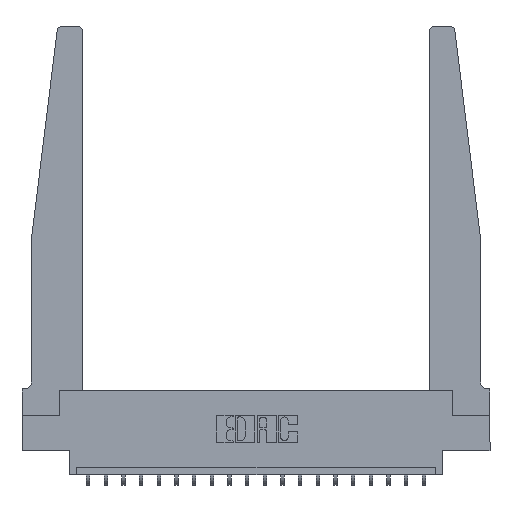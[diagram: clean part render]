
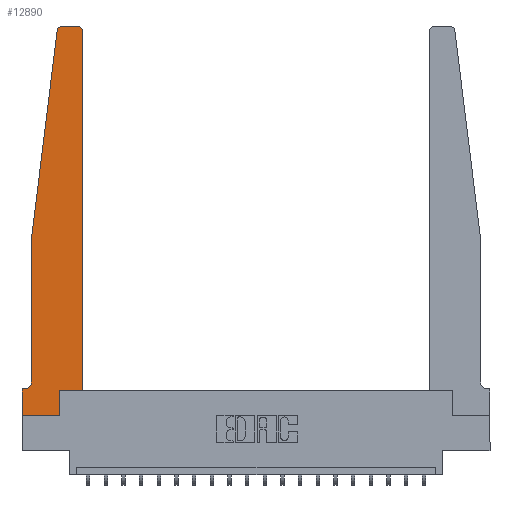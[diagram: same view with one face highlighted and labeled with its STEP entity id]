
A CAD part, top view. The second image highlights one B-rep face of the part: STEP entity #12890.
In plain terms, the highlighted planar face has unit normal (0, 0, 1).
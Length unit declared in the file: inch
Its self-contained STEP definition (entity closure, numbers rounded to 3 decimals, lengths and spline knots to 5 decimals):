
#287 = VECTOR ( 'NONE', #11607, 39.37008 ) ;
#391 = EDGE_CURVE ( 'NONE', #1555, #17705, #18310, .T. ) ;
#419 = LINE ( 'NONE', #6538, #4378 ) ;
#451 = DIRECTION ( 'NONE',  ( -1., 0., 0. ) ) ;
#769 = CARTESIAN_POINT ( 'NONE',  ( 0.395, 2.72, 0.37 ) ) ;
#806 = CARTESIAN_POINT ( 'NONE',  ( 0.2605, 0.18, 0.37 ) ) ;
#809 = EDGE_CURVE ( 'NONE', #17705, #7202, #2419, .T. ) ;
#1295 = LINE ( 'NONE', #3190, #1606 ) ;
#1555 = VERTEX_POINT ( 'NONE', #19395 ) ;
#1606 = VECTOR ( 'NONE', #17604, 39.37008 ) ;
#1727 = CARTESIAN_POINT ( 'NONE',  ( 0., 0.1875, 0.37 ) ) ;
#1750 = CARTESIAN_POINT ( 'NONE',  ( 0.015, 0.1875, 0.37 ) ) ;
#1813 = ORIENTED_EDGE ( 'NONE', *, *, #809, .T. ) ;
#2112 = DIRECTION ( 'NONE',  ( -1., 0., 0. ) ) ;
#2259 = CARTESIAN_POINT ( 'NONE',  ( 0.425, 2.72, 0.37 ) ) ;
#2419 = LINE ( 'NONE', #16705, #19772 ) ;
#3012 = EDGE_LOOP ( 'NONE', ( #16483, #19728, #16349, #1813, #17590, #5781, #17220, #20670, #18151, #8635, #3396, #18256 ) ) ;
#3190 = CARTESIAN_POINT ( 'NONE',  ( 0., 0., 0.37 ) ) ;
#3396 = ORIENTED_EDGE ( 'NONE', *, *, #15649, .T. ) ;
#3664 = CARTESIAN_POINT ( 'NONE',  ( 0.425, 0.18, 0.37 ) ) ;
#3763 = DIRECTION ( 'NONE',  ( 0., 0., 1. ) ) ;
#3766 = VERTEX_POINT ( 'NONE', #19923 ) ;
#4326 = DIRECTION ( 'NONE',  ( 0., 1., 0. ) ) ;
#4370 = CARTESIAN_POINT ( 'NONE',  ( 0.2605, 0.18, 0.37 ) ) ;
#4378 = VECTOR ( 'NONE', #2112, 39.37008 ) ;
#4494 = CARTESIAN_POINT ( 'NONE',  ( 0.015, 0.2375, 0.37 ) ) ;
#4539 = AXIS2_PLACEMENT_3D ( 'NONE', #9388, #11543, #19548 ) ;
#4913 = VERTEX_POINT ( 'NONE', #15503 ) ;
#4918 = VECTOR ( 'NONE', #8420, 39.37008 ) ;
#5444 = EDGE_CURVE ( 'NONE', #6255, #16433, #419, .T. ) ;
#5508 = CARTESIAN_POINT ( 'NONE',  ( 0.065, 1.25, 0.37 ) ) ;
#5580 = LINE ( 'NONE', #15124, #4918 ) ;
#5781 = ORIENTED_EDGE ( 'NONE', *, *, #5444, .T. ) ;
#5790 = VECTOR ( 'NONE', #8516, 39.37008 ) ;
#5937 = EDGE_CURVE ( 'NONE', #8788, #1555, #10080, .T. ) ;
#6122 = LINE ( 'NONE', #10741, #7025 ) ;
#6255 = VERTEX_POINT ( 'NONE', #1750 ) ;
#6275 = CARTESIAN_POINT ( 'NONE',  ( 0.065, 1.25, 0.37 ) ) ;
#6538 = CARTESIAN_POINT ( 'NONE',  ( 0.065, 0.1875, 0.37 ) ) ;
#6675 = EDGE_CURVE ( 'NONE', #16186, #20377, #12106, .T. ) ;
#6851 = FACE_OUTER_BOUND ( 'NONE', #3012, .T. ) ;
#7025 = VECTOR ( 'NONE', #4326, 39.37008 ) ;
#7202 = VERTEX_POINT ( 'NONE', #18635 ) ;
#7243 = CARTESIAN_POINT ( 'NONE',  ( 0.27653, 2.72, 0.37 ) ) ;
#7995 = EDGE_CURVE ( 'NONE', #12385, #4913, #18066, .T. ) ;
#8420 = DIRECTION ( 'NONE',  ( 0., -1., 0. ) ) ;
#8437 = CARTESIAN_POINT ( 'NONE',  ( 0.395, 2.75, 0.37 ) ) ;
#8516 = DIRECTION ( 'NONE',  ( 1., 0., 0. ) ) ;
#8635 = ORIENTED_EDGE ( 'NONE', *, *, #7995, .T. ) ;
#8788 = VERTEX_POINT ( 'NONE', #18329 ) ;
#9281 = CARTESIAN_POINT ( 'NONE',  ( 0.2605, 0., 0.37 ) ) ;
#9388 = CARTESIAN_POINT ( 'NONE',  ( 0., 0.1875, 0.37 ) ) ;
#10080 = CIRCLE ( 'NONE', #18142, 0.03 ) ;
#10436 = DIRECTION ( 'NONE',  ( -0.122, -0.992, 0. ) ) ;
#10741 = CARTESIAN_POINT ( 'NONE',  ( 0.425, 0.18, 0.37 ) ) ;
#11082 = VERTEX_POINT ( 'NONE', #9281 ) ;
#11543 = DIRECTION ( 'NONE',  ( 0., 0., 1. ) ) ;
#11607 = DIRECTION ( 'NONE',  ( -1., 0., 0. ) ) ;
#11664 = VECTOR ( 'NONE', #10436, 39.37008 ) ;
#11689 = DIRECTION ( 'NONE',  ( 0., 0., 1. ) ) ;
#12106 = CIRCLE ( 'NONE', #16835, 0.03 ) ;
#12385 = VERTEX_POINT ( 'NONE', #4370 ) ;
#12890 = ADVANCED_FACE ( 'NONE', ( #6851 ), #19751, .T. ) ;
#13372 = DIRECTION ( 'NONE',  ( 1., 0., 0. ) ) ;
#13417 = EDGE_CURVE ( 'NONE', #11082, #12385, #19724, .T. ) ;
#13548 = DIRECTION ( 'NONE',  ( 0., -1., 0. ) ) ;
#14740 = EDGE_CURVE ( 'NONE', #16433, #3766, #5580, .T. ) ;
#15124 = CARTESIAN_POINT ( 'NONE',  ( 0., 0., 0.37 ) ) ;
#15503 = CARTESIAN_POINT ( 'NONE',  ( 0.425, 0.18, 0.37 ) ) ;
#15649 = EDGE_CURVE ( 'NONE', #4913, #16186, #6122, .T. ) ;
#16146 = LINE ( 'NONE', #19300, #287 ) ;
#16186 = VERTEX_POINT ( 'NONE', #2259 ) ;
#16349 = ORIENTED_EDGE ( 'NONE', *, *, #391, .T. ) ;
#16433 = VERTEX_POINT ( 'NONE', #1727 ) ;
#16483 = ORIENTED_EDGE ( 'NONE', *, *, #17805, .T. ) ;
#16542 = EDGE_CURVE ( 'NONE', #3766, #11082, #1295, .T. ) ;
#16705 = CARTESIAN_POINT ( 'NONE',  ( 0.065, 1.25, 0.37 ) ) ;
#16835 = AXIS2_PLACEMENT_3D ( 'NONE', #769, #11689, #13372 ) ;
#17220 = ORIENTED_EDGE ( 'NONE', *, *, #14740, .T. ) ;
#17307 = DIRECTION ( 'NONE',  ( 0., 0., -1. ) ) ;
#17590 = ORIENTED_EDGE ( 'NONE', *, *, #19909, .T. ) ;
#17604 = DIRECTION ( 'NONE',  ( 1., 0., 0. ) ) ;
#17705 = VERTEX_POINT ( 'NONE', #6275 ) ;
#17805 = EDGE_CURVE ( 'NONE', #20377, #8788, #16146, .T. ) ;
#17981 = VECTOR ( 'NONE', #20039, 39.37008 ) ;
#18066 = LINE ( 'NONE', #3664, #5790 ) ;
#18142 = AXIS2_PLACEMENT_3D ( 'NONE', #7243, #3763, #19950 ) ;
#18151 = ORIENTED_EDGE ( 'NONE', *, *, #13417, .T. ) ;
#18256 = ORIENTED_EDGE ( 'NONE', *, *, #6675, .T. ) ;
#18310 = LINE ( 'NONE', #5508, #11664 ) ;
#18329 = CARTESIAN_POINT ( 'NONE',  ( 0.27653, 2.75, 0.37 ) ) ;
#18635 = CARTESIAN_POINT ( 'NONE',  ( 0.065, 0.2375, 0.37 ) ) ;
#19121 = CIRCLE ( 'NONE', #20130, 0.05 ) ;
#19300 = CARTESIAN_POINT ( 'NONE',  ( 0.25, 2.75, 0.37 ) ) ;
#19395 = CARTESIAN_POINT ( 'NONE',  ( 0.24675, 2.72367, 0.37 ) ) ;
#19548 = DIRECTION ( 'NONE',  ( 1., 0., 0. ) ) ;
#19724 = LINE ( 'NONE', #806, #17981 ) ;
#19728 = ORIENTED_EDGE ( 'NONE', *, *, #5937, .T. ) ;
#19751 = PLANE ( 'NONE',  #4539 ) ;
#19772 = VECTOR ( 'NONE', #13548, 39.37008 ) ;
#19909 = EDGE_CURVE ( 'NONE', #7202, #6255, #19121, .T. ) ;
#19923 = CARTESIAN_POINT ( 'NONE',  ( 0., 0., 0.37 ) ) ;
#19950 = DIRECTION ( 'NONE',  ( 1., 0., 0. ) ) ;
#20039 = DIRECTION ( 'NONE',  ( 0., 1., 0. ) ) ;
#20130 = AXIS2_PLACEMENT_3D ( 'NONE', #4494, #17307, #451 ) ;
#20377 = VERTEX_POINT ( 'NONE', #8437 ) ;
#20670 = ORIENTED_EDGE ( 'NONE', *, *, #16542, .T. ) ;
